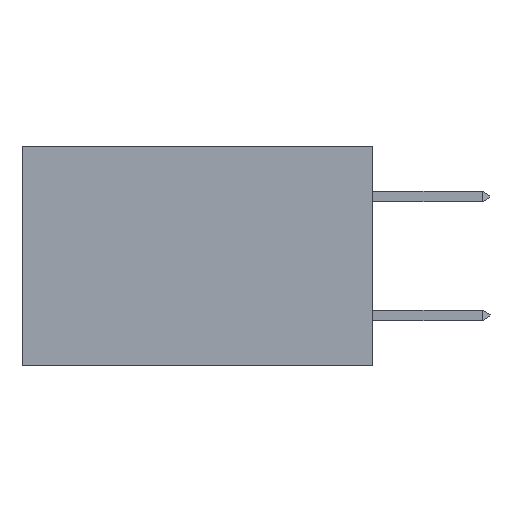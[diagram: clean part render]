
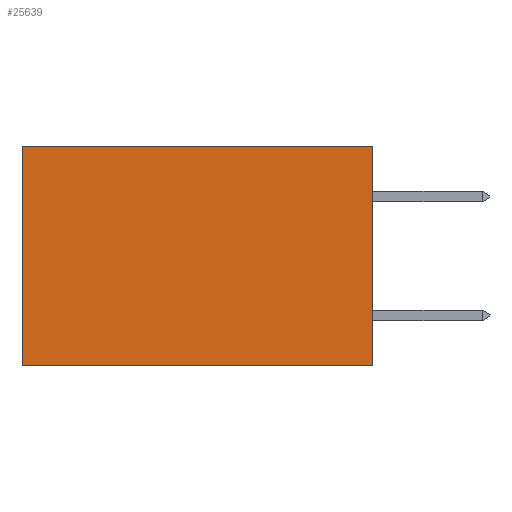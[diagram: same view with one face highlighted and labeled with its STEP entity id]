
A CAD part, left-side view. The second image highlights one B-rep face of the part: STEP entity #25639.
In plain terms, the highlighted planar face has unit normal (-1, 0, 0).
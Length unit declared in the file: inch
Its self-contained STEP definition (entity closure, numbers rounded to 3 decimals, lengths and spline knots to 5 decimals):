
#665 = LINE ( 'NONE', #23466, #21052 ) ;
#1300 = CARTESIAN_POINT ( 'NONE',  ( 0.277, 0., 0. ) ) ;
#1585 = ORIENTED_EDGE ( 'NONE', *, *, #16917, .T. ) ;
#1889 = VECTOR ( 'NONE', #32529, 39.37008 ) ;
#2925 = CARTESIAN_POINT ( 'NONE',  ( 0.277, 0., 0. ) ) ;
#3403 = ORIENTED_EDGE ( 'NONE', *, *, #25411, .T. ) ;
#3600 = CARTESIAN_POINT ( 'NONE',  ( 0.277, 0.59, -0.37 ) ) ;
#3850 = DIRECTION ( 'NONE',  ( 0., 1., 0. ) ) ;
#4529 = PLANE ( 'NONE',  #14657 ) ;
#7660 = VERTEX_POINT ( 'NONE', #2925 ) ;
#8557 = VECTOR ( 'NONE', #3850, 39.37008 ) ;
#8638 = FACE_OUTER_BOUND ( 'NONE', #25483, .T. ) ;
#8703 = DIRECTION ( 'NONE',  ( 0., 0., -1. ) ) ;
#10852 = VERTEX_POINT ( 'NONE', #30010 ) ;
#13272 = DIRECTION ( 'NONE',  ( 0., 1., 0. ) ) ;
#14657 = AXIS2_PLACEMENT_3D ( 'NONE', #19947, #14883, #32630 ) ;
#14883 = DIRECTION ( 'NONE',  ( 1., 0., 0. ) ) ;
#16917 = EDGE_CURVE ( 'NONE', #24901, #10852, #26831, .T. ) ;
#18397 = ORIENTED_EDGE ( 'NONE', *, *, #25618, .F. ) ;
#19947 = CARTESIAN_POINT ( 'NONE',  ( 0.277, 0., -0.37 ) ) ;
#20789 = VERTEX_POINT ( 'NONE', #30335 ) ;
#21052 = VECTOR ( 'NONE', #13272, 39.37008 ) ;
#22246 = LINE ( 'NONE', #30005, #1889 ) ;
#23466 = CARTESIAN_POINT ( 'NONE',  ( 0.277, 0., -0.37 ) ) ;
#24901 = VERTEX_POINT ( 'NONE', #30043 ) ;
#25411 = EDGE_CURVE ( 'NONE', #7660, #24901, #28897, .T. ) ;
#25483 = EDGE_LOOP ( 'NONE', ( #1585, #25721, #18397, #3403 ) ) ;
#25618 = EDGE_CURVE ( 'NONE', #7660, #20789, #22246, .T. ) ;
#25639 = ADVANCED_FACE ( 'NONE', ( #8638 ), #4529, .F. ) ;
#25721 = ORIENTED_EDGE ( 'NONE', *, *, #25902, .F. ) ;
#25902 = EDGE_CURVE ( 'NONE', #20789, #10852, #665, .T. ) ;
#26831 = LINE ( 'NONE', #3600, #32736 ) ;
#28897 = LINE ( 'NONE', #1300, #8557 ) ;
#30005 = CARTESIAN_POINT ( 'NONE',  ( 0.277, 0., -0.37 ) ) ;
#30010 = CARTESIAN_POINT ( 'NONE',  ( 0.277, 0.59, -0.37 ) ) ;
#30043 = CARTESIAN_POINT ( 'NONE',  ( 0.277, 0.59, 0. ) ) ;
#30335 = CARTESIAN_POINT ( 'NONE',  ( 0.277, 0., -0.37 ) ) ;
#32529 = DIRECTION ( 'NONE',  ( 0., 0., -1. ) ) ;
#32630 = DIRECTION ( 'NONE',  ( 0., 0., -1. ) ) ;
#32736 = VECTOR ( 'NONE', #8703, 39.37008 ) ;
